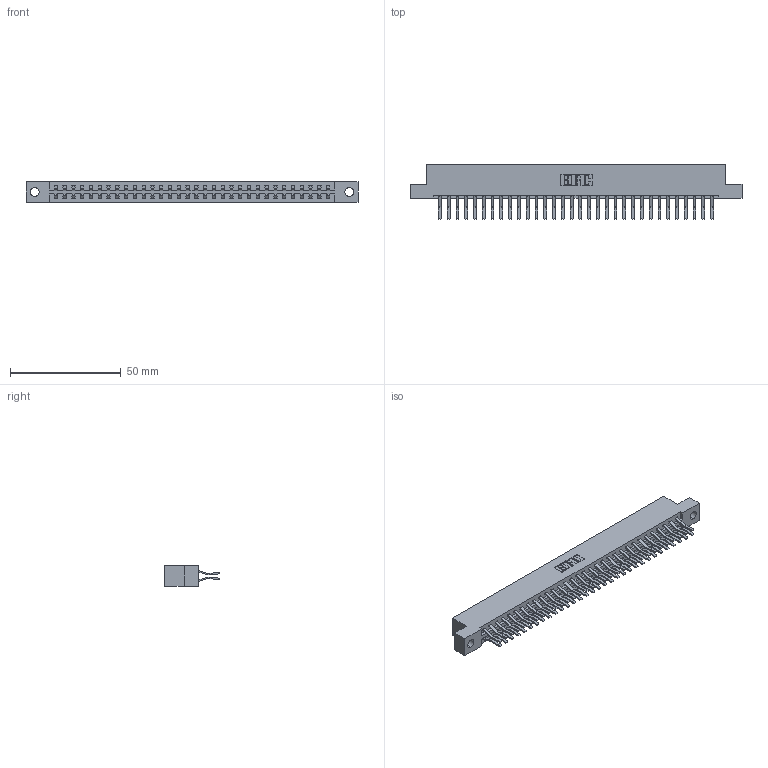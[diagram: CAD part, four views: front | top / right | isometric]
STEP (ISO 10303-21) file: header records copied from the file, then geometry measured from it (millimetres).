
FILE_DESCRIPTION (( 'STEP AP203' ), '1' );
FILE_NAME ('337-064-560-204.STEP', '2019-10-09T22:44:05', ( '' ), ( '' ), 'SwSTEP 2.0', 'SolidWorks 2016', '' );
FILE_SCHEMA (( 'CONFIG_CONTROL_DESIGN' ));
Length unit declared in the file: inch
Products named in the file (3): 345-292-001_560 Tail; 337-064-560-204; 337 Part_Flush Mounting Lugs - 0.156 Dia-TH
Assembly tree (65 placements, depth 2):
  337-064-560-204
    337 Part_Flush Mounting Lugs - 0.156 Dia-TH
    345-292-001_560 Tail  x64
Bounding box: 149.81 x 24.78 x 9.4 mm (x, y, z)
Volume: 15986.6 mm3; surface area: 18987.3 mm2
Topology: 65 solids, 65 shells, 3698 faces, 10999 edges, 7246 vertices
Faces by surface type: plane 2502, cylinder 1196
Entity records: 26195 total; most frequent: CARTESIAN_POINT 4422, ORIENTED_EDGE 4358, DIRECTION 3783, EDGE_CURVE 2179, LINE 2047, VECTOR 2047, VERTEX_POINT 1450, AXIS2_PLACEMENT_3D 868
